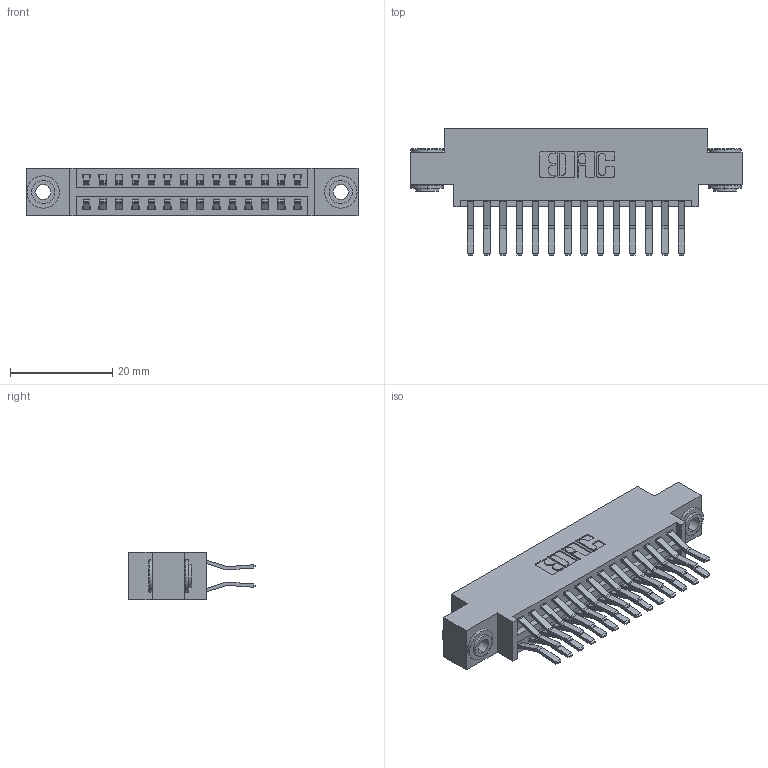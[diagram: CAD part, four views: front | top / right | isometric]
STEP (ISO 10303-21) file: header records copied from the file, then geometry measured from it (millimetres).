
FILE_DESCRIPTION (( 'STEP AP203' ), '1' );
FILE_NAME ('346-028-560-803.STEP', '2018-08-22T02:49:59', ( '' ), ( '' ), 'SwSTEP 2.0', 'SolidWorks 2016', '' );
FILE_SCHEMA (( 'CONFIG_CONTROL_DESIGN' ));
Length unit declared in the file: inch
Products named in the file (4): 346-028-560-803; 346 Part_0.170 Offset - 0.156 Dia-TH; 345-292-001_560 Tail; 345-250-002_345-250-002-102
Assembly tree (31 placements, depth 2):
  346-028-560-803
    346 Part_0.170 Offset - 0.156 Dia-TH
    345-292-001_560 Tail  x28
    345-250-002_345-250-002-102  x2
Bounding box: 65.02 x 24.78 x 9.4 mm (x, y, z)
Volume: 6171.5 mm3; surface area: 8926.5 mm2
Topology: 31 solids, 31 shells, 1676 faces, 4925 edges, 3242 vertices
Faces by surface type: plane 1070, cylinder 598, cone 8
Entity records: 13776 total; most frequent: CARTESIAN_POINT 2287, ORIENTED_EDGE 2214, DIRECTION 2101, EDGE_CURVE 1107, VECTOR 891, LINE 891, VERTEX_POINT 734, AXIS2_PLACEMENT_3D 605
